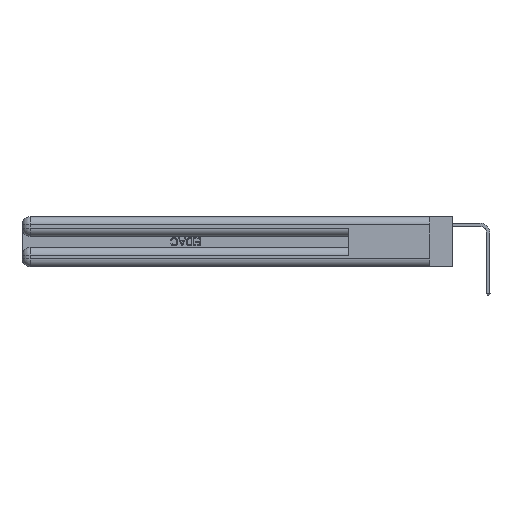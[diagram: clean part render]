
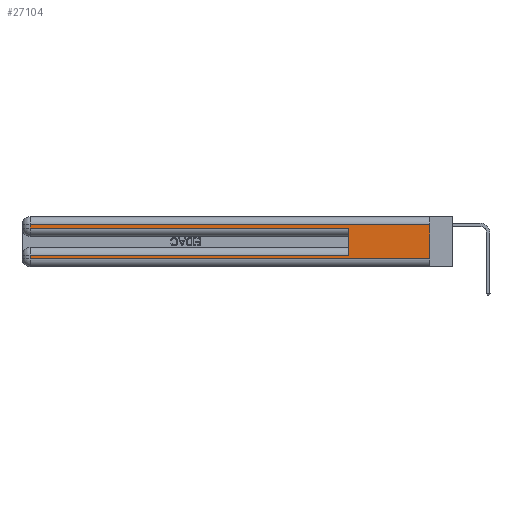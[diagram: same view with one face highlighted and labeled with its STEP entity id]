
A CAD part, left-side view. The second image highlights one B-rep face of the part: STEP entity #27104.
In plain terms, the highlighted planar face has unit normal (-1, 0, 0).
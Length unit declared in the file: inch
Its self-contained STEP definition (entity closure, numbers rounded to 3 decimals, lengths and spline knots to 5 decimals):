
#201 = DIRECTION ( 'NONE',  ( 0., 0., -1. ) ) ;
#1191 = LINE ( 'NONE', #5749, #20257 ) ;
#1382 = ORIENTED_EDGE ( 'NONE', *, *, #25347, .F. ) ;
#1450 = VERTEX_POINT ( 'NONE', #5408 ) ;
#1805 = VERTEX_POINT ( 'NONE', #16819 ) ;
#1928 = DIRECTION ( 'NONE',  ( 0., 0., 1. ) ) ;
#2223 = DIRECTION ( 'NONE',  ( 0., -1., 0. ) ) ;
#2987 = VERTEX_POINT ( 'NONE', #26331 ) ;
#3343 = VECTOR ( 'NONE', #6952, 39.37008 ) ;
#3387 = DIRECTION ( 'NONE',  ( 0., 0., -1. ) ) ;
#3846 = LINE ( 'NONE', #25587, #10697 ) ;
#3850 = DIRECTION ( 'NONE',  ( 0., 0., -1. ) ) ;
#4177 = CARTESIAN_POINT ( 'NONE',  ( 0., 2.94, 0.31 ) ) ;
#4409 = LINE ( 'NONE', #23490, #3343 ) ;
#4914 = FACE_OUTER_BOUND ( 'NONE', #26097, .T. ) ;
#5188 = ORIENTED_EDGE ( 'NONE', *, *, #18334, .T. ) ;
#5408 = CARTESIAN_POINT ( 'NONE',  ( 0., 0.6, 0.285 ) ) ;
#5749 = CARTESIAN_POINT ( 'NONE',  ( 0., 2.94, 0.37 ) ) ;
#6017 = ORIENTED_EDGE ( 'NONE', *, *, #14930, .T. ) ;
#6218 = LINE ( 'NONE', #15762, #27616 ) ;
#6793 = EDGE_CURVE ( 'NONE', #14706, #22911, #4409, .T. ) ;
#6952 = DIRECTION ( 'NONE',  ( 0., 1., 0. ) ) ;
#7260 = LINE ( 'NONE', #11822, #23400 ) ;
#7451 = DIRECTION ( 'NONE',  ( 1., 0., 0. ) ) ;
#7563 = CARTESIAN_POINT ( 'NONE',  ( 0., 0.6, 0.085 ) ) ;
#8082 = EDGE_CURVE ( 'NONE', #2987, #1450, #7260, .T. ) ;
#9426 = VECTOR ( 'NONE', #17006, 39.37008 ) ;
#10697 = VECTOR ( 'NONE', #16074, 39.37008 ) ;
#11822 = CARTESIAN_POINT ( 'NONE',  ( 0., 0., 0.285 ) ) ;
#14527 = CARTESIAN_POINT ( 'NONE',  ( 0., 0., 0.37 ) ) ;
#14645 = PLANE ( 'NONE',  #22329 ) ;
#14706 = VERTEX_POINT ( 'NONE', #22007 ) ;
#14930 = EDGE_CURVE ( 'NONE', #22911, #2987, #6218, .T. ) ;
#15404 = LINE ( 'NONE', #18035, #27814 ) ;
#15762 = CARTESIAN_POINT ( 'NONE',  ( 0., 2.94, 0.37 ) ) ;
#16074 = DIRECTION ( 'NONE',  ( 0., 1., 0. ) ) ;
#16790 = VERTEX_POINT ( 'NONE', #28455 ) ;
#16819 = CARTESIAN_POINT ( 'NONE',  ( 0., 2.94, 0.085 ) ) ;
#17006 = DIRECTION ( 'NONE',  ( 0., 0., -1. ) ) ;
#17110 = ORIENTED_EDGE ( 'NONE', *, *, #6793, .T. ) ;
#18035 = CARTESIAN_POINT ( 'NONE',  ( 0., 0., 0.06 ) ) ;
#18280 = VECTOR ( 'NONE', #1928, 39.37008 ) ;
#18293 = CARTESIAN_POINT ( 'NONE',  ( 0., 2.94, 0.06 ) ) ;
#18334 = EDGE_CURVE ( 'NONE', #21142, #1805, #3846, .T. ) ;
#19010 = CARTESIAN_POINT ( 'NONE',  ( 0., 0., 0.37 ) ) ;
#20257 = VECTOR ( 'NONE', #3387, 39.37008 ) ;
#21142 = VERTEX_POINT ( 'NONE', #7563 ) ;
#22007 = CARTESIAN_POINT ( 'NONE',  ( 0., 0., 0.31 ) ) ;
#22102 = ORIENTED_EDGE ( 'NONE', *, *, #8082, .T. ) ;
#22329 = AXIS2_PLACEMENT_3D ( 'NONE', #19010, #7451, #201 ) ;
#22911 = VERTEX_POINT ( 'NONE', #4177 ) ;
#23240 = EDGE_CURVE ( 'NONE', #1805, #28764, #1191, .T. ) ;
#23400 = VECTOR ( 'NONE', #2223, 39.37008 ) ;
#23490 = CARTESIAN_POINT ( 'NONE',  ( 0., 0., 0.31 ) ) ;
#23726 = EDGE_CURVE ( 'NONE', #21142, #1450, #25701, .T. ) ;
#24222 = EDGE_CURVE ( 'NONE', #28764, #16790, #15404, .T. ) ;
#25347 = EDGE_CURVE ( 'NONE', #14706, #16790, #28588, .T. ) ;
#25388 = CARTESIAN_POINT ( 'NONE',  ( 0., 0.6, 0.145 ) ) ;
#25587 = CARTESIAN_POINT ( 'NONE',  ( 0., 0., 0.085 ) ) ;
#25701 = LINE ( 'NONE', #25388, #18280 ) ;
#26097 = EDGE_LOOP ( 'NONE', ( #1382, #17110, #6017, #22102, #28538, #5188, #28290, #27319 ) ) ;
#26331 = CARTESIAN_POINT ( 'NONE',  ( 0., 2.94, 0.285 ) ) ;
#27098 = DIRECTION ( 'NONE',  ( 0., -1., 0. ) ) ;
#27104 = ADVANCED_FACE ( 'NONE', ( #4914 ), #14645, .F. ) ;
#27319 = ORIENTED_EDGE ( 'NONE', *, *, #24222, .T. ) ;
#27616 = VECTOR ( 'NONE', #3850, 39.37008 ) ;
#27814 = VECTOR ( 'NONE', #27098, 39.37008 ) ;
#28290 = ORIENTED_EDGE ( 'NONE', *, *, #23240, .T. ) ;
#28455 = CARTESIAN_POINT ( 'NONE',  ( 0., 0., 0.06 ) ) ;
#28538 = ORIENTED_EDGE ( 'NONE', *, *, #23726, .F. ) ;
#28588 = LINE ( 'NONE', #14527, #9426 ) ;
#28764 = VERTEX_POINT ( 'NONE', #18293 ) ;
